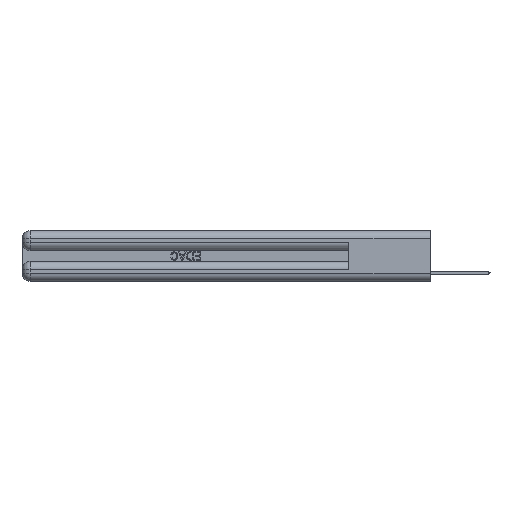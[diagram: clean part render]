
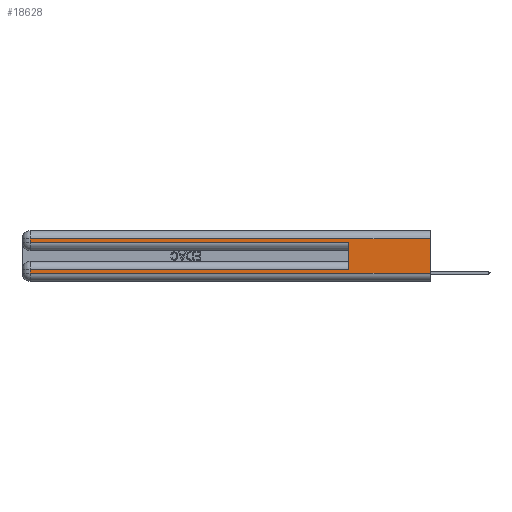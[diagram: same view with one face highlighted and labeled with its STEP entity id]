
A CAD part, left-side view. The second image highlights one B-rep face of the part: STEP entity #18628.
In plain terms, the highlighted planar face has unit normal (-1, 0, 0).
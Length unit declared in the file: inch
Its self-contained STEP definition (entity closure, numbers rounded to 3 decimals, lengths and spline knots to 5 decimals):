
#5 = CARTESIAN_POINT ( 'NONE',  ( 0., 0., 0.37 ) ) ;
#1170 = LINE ( 'NONE', #11667, #4894 ) ;
#1717 = CARTESIAN_POINT ( 'NONE',  ( 0., 0.6, 0.285 ) ) ;
#2463 = LINE ( 'NONE', #10805, #19900 ) ;
#2492 = DIRECTION ( 'NONE',  ( 0., 0., -1. ) ) ;
#2641 = CARTESIAN_POINT ( 'NONE',  ( 0., 0., 0.31 ) ) ;
#3136 = VERTEX_POINT ( 'NONE', #14344 ) ;
#3546 = VECTOR ( 'NONE', #19593, 39.37008 ) ;
#4264 = EDGE_LOOP ( 'NONE', ( #11468, #22986, #12234, #15092, #31182, #15387, #29057, #5468 ) ) ;
#4894 = VECTOR ( 'NONE', #19326, 39.37008 ) ;
#5468 = ORIENTED_EDGE ( 'NONE', *, *, #29473, .T. ) ;
#5512 = VECTOR ( 'NONE', #13741, 39.37008 ) ;
#6040 = VERTEX_POINT ( 'NONE', #29682 ) ;
#6514 = VERTEX_POINT ( 'NONE', #26520 ) ;
#6602 = EDGE_CURVE ( 'NONE', #6040, #10611, #1170, .T. ) ;
#7386 = EDGE_CURVE ( 'NONE', #6040, #6514, #15836, .T. ) ;
#7733 = VERTEX_POINT ( 'NONE', #21444 ) ;
#7746 = VERTEX_POINT ( 'NONE', #9343 ) ;
#7755 = AXIS2_PLACEMENT_3D ( 'NONE', #5, #21578, #14361 ) ;
#8231 = VECTOR ( 'NONE', #28112, 39.37008 ) ;
#9343 = CARTESIAN_POINT ( 'NONE',  ( 0., 2.94, 0.06 ) ) ;
#10528 = EDGE_CURVE ( 'NONE', #16058, #7733, #30243, .T. ) ;
#10611 = VERTEX_POINT ( 'NONE', #1717 ) ;
#10805 = CARTESIAN_POINT ( 'NONE',  ( 0., 2.94, 0.37 ) ) ;
#11468 = ORIENTED_EDGE ( 'NONE', *, *, #10528, .F. ) ;
#11495 = CARTESIAN_POINT ( 'NONE',  ( 0., 0., 0.285 ) ) ;
#11667 = CARTESIAN_POINT ( 'NONE',  ( 0., 0.6, 0.145 ) ) ;
#12234 = ORIENTED_EDGE ( 'NONE', *, *, #27794, .T. ) ;
#13741 = DIRECTION ( 'NONE',  ( 0., -1., 0. ) ) ;
#13917 = EDGE_CURVE ( 'NONE', #6514, #7746, #2463, .T. ) ;
#14344 = CARTESIAN_POINT ( 'NONE',  ( 0., 2.94, 0.285 ) ) ;
#14361 = DIRECTION ( 'NONE',  ( 0., 0., -1. ) ) ;
#14847 = FACE_OUTER_BOUND ( 'NONE', #4264, .T. ) ;
#15092 = ORIENTED_EDGE ( 'NONE', *, *, #27193, .T. ) ;
#15254 = VECTOR ( 'NONE', #21234, 39.37008 ) ;
#15387 = ORIENTED_EDGE ( 'NONE', *, *, #7386, .T. ) ;
#15719 = VERTEX_POINT ( 'NONE', #21615 ) ;
#15836 = LINE ( 'NONE', #26896, #8231 ) ;
#16036 = LINE ( 'NONE', #29374, #3546 ) ;
#16058 = VERTEX_POINT ( 'NONE', #2641 ) ;
#16601 = PLANE ( 'NONE',  #7755 ) ;
#18628 = ADVANCED_FACE ( 'NONE', ( #14847 ), #16601, .F. ) ;
#19326 = DIRECTION ( 'NONE',  ( 0., 0., 1. ) ) ;
#19593 = DIRECTION ( 'NONE',  ( 0., 1., 0. ) ) ;
#19900 = VECTOR ( 'NONE', #20377, 39.37008 ) ;
#19947 = LINE ( 'NONE', #11495, #5512 ) ;
#20377 = DIRECTION ( 'NONE',  ( 0., 0., -1. ) ) ;
#21234 = DIRECTION ( 'NONE',  ( 0., -1., 0. ) ) ;
#21444 = CARTESIAN_POINT ( 'NONE',  ( 0., 0., 0.06 ) ) ;
#21578 = DIRECTION ( 'NONE',  ( 1., 0., 0. ) ) ;
#21615 = CARTESIAN_POINT ( 'NONE',  ( 0., 2.94, 0.31 ) ) ;
#22160 = CARTESIAN_POINT ( 'NONE',  ( 0., 2.94, 0.37 ) ) ;
#22986 = ORIENTED_EDGE ( 'NONE', *, *, #28539, .T. ) ;
#23079 = CARTESIAN_POINT ( 'NONE',  ( 0., 0., 0.37 ) ) ;
#23272 = VECTOR ( 'NONE', #2492, 39.37008 ) ;
#25499 = DIRECTION ( 'NONE',  ( 0., 0., -1. ) ) ;
#26520 = CARTESIAN_POINT ( 'NONE',  ( 0., 2.94, 0.085 ) ) ;
#26896 = CARTESIAN_POINT ( 'NONE',  ( 0., 0., 0.085 ) ) ;
#27193 = EDGE_CURVE ( 'NONE', #3136, #10611, #19947, .T. ) ;
#27794 = EDGE_CURVE ( 'NONE', #15719, #3136, #28156, .T. ) ;
#28068 = LINE ( 'NONE', #28784, #15254 ) ;
#28112 = DIRECTION ( 'NONE',  ( 0., 1., 0. ) ) ;
#28156 = LINE ( 'NONE', #22160, #23272 ) ;
#28539 = EDGE_CURVE ( 'NONE', #16058, #15719, #16036, .T. ) ;
#28784 = CARTESIAN_POINT ( 'NONE',  ( 0., 0., 0.06 ) ) ;
#29057 = ORIENTED_EDGE ( 'NONE', *, *, #13917, .T. ) ;
#29374 = CARTESIAN_POINT ( 'NONE',  ( 0., 0., 0.31 ) ) ;
#29473 = EDGE_CURVE ( 'NONE', #7746, #7733, #28068, .T. ) ;
#29486 = VECTOR ( 'NONE', #25499, 39.37008 ) ;
#29682 = CARTESIAN_POINT ( 'NONE',  ( 0., 0.6, 0.085 ) ) ;
#30243 = LINE ( 'NONE', #23079, #29486 ) ;
#31182 = ORIENTED_EDGE ( 'NONE', *, *, #6602, .F. ) ;
